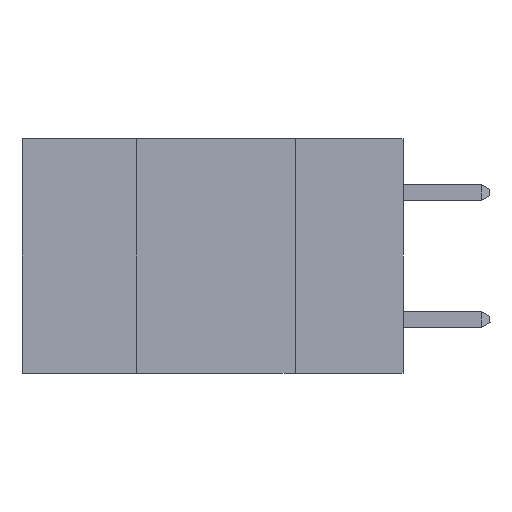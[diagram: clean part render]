
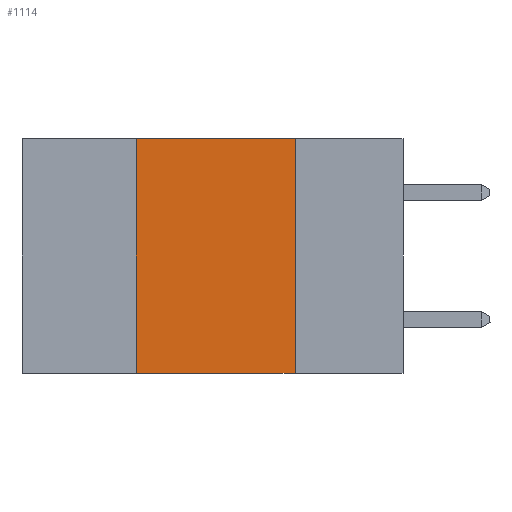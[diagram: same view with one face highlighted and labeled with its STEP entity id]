
A CAD part, left-side view. The second image highlights one B-rep face of the part: STEP entity #1114.
In plain terms, the highlighted planar face has unit normal (-1, 0, 0).
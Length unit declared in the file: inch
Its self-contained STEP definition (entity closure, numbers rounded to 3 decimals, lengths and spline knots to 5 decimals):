
#191 = LINE ( 'NONE', #6273, #8206 ) ;
#253 = ORIENTED_EDGE ( 'NONE', *, *, #9417, .T. ) ;
#265 = LINE ( 'NONE', #1840, #527 ) ;
#527 = VECTOR ( 'NONE', #1000, 39.37008 ) ;
#975 = LINE ( 'NONE', #8532, #9134 ) ;
#1000 = DIRECTION ( 'NONE',  ( 0., -1., 0. ) ) ;
#1114 = ADVANCED_FACE ( 'NONE', ( #8581 ), #5776, .F. ) ;
#1609 = CARTESIAN_POINT ( 'NONE',  ( 0., 0.17, -0.37 ) ) ;
#1635 = CARTESIAN_POINT ( 'NONE',  ( 0., 0.6, 0. ) ) ;
#1840 = CARTESIAN_POINT ( 'NONE',  ( 0., 0.6, 0. ) ) ;
#1849 = EDGE_CURVE ( 'NONE', #6471, #5223, #191, .T. ) ;
#2666 = CARTESIAN_POINT ( 'NONE',  ( 0., 0.6, -0.37 ) ) ;
#2683 = CARTESIAN_POINT ( 'NONE',  ( 0., 0.42, -0.37 ) ) ;
#3032 = DIRECTION ( 'NONE',  ( 0., 0., -1. ) ) ;
#3168 = EDGE_CURVE ( 'NONE', #5223, #5519, #265, .T. ) ;
#3614 = CARTESIAN_POINT ( 'NONE',  ( 0., 0.42, 0. ) ) ;
#3708 = DIRECTION ( 'NONE',  ( 0., 0., -1. ) ) ;
#4858 = ORIENTED_EDGE ( 'NONE', *, *, #1849, .F. ) ;
#5223 = VERTEX_POINT ( 'NONE', #3614 ) ;
#5519 = VERTEX_POINT ( 'NONE', #6344 ) ;
#5557 = VERTEX_POINT ( 'NONE', #1609 ) ;
#5776 = PLANE ( 'NONE',  #10204 ) ;
#5927 = LINE ( 'NONE', #2666, #7733 ) ;
#5986 = EDGE_LOOP ( 'NONE', ( #8961, #7073, #4858, #253 ) ) ;
#6273 = CARTESIAN_POINT ( 'NONE',  ( 0., 0.42, 0. ) ) ;
#6344 = CARTESIAN_POINT ( 'NONE',  ( 0., 0.17, 0. ) ) ;
#6471 = VERTEX_POINT ( 'NONE', #2683 ) ;
#7073 = ORIENTED_EDGE ( 'NONE', *, *, #3168, .F. ) ;
#7733 = VECTOR ( 'NONE', #8171, 39.37008 ) ;
#7867 = EDGE_CURVE ( 'NONE', #5519, #5557, #975, .T. ) ;
#8171 = DIRECTION ( 'NONE',  ( 0., -1., 0. ) ) ;
#8206 = VECTOR ( 'NONE', #8912, 39.37008 ) ;
#8532 = CARTESIAN_POINT ( 'NONE',  ( 0., 0.17, 0. ) ) ;
#8581 = FACE_OUTER_BOUND ( 'NONE', #5986, .T. ) ;
#8912 = DIRECTION ( 'NONE',  ( 0., 0., 1. ) ) ;
#8961 = ORIENTED_EDGE ( 'NONE', *, *, #7867, .F. ) ;
#9134 = VECTOR ( 'NONE', #3032, 39.37008 ) ;
#9229 = DIRECTION ( 'NONE',  ( 1., 0., 0. ) ) ;
#9417 = EDGE_CURVE ( 'NONE', #6471, #5557, #5927, .T. ) ;
#10204 = AXIS2_PLACEMENT_3D ( 'NONE', #1635, #9229, #3708 ) ;
